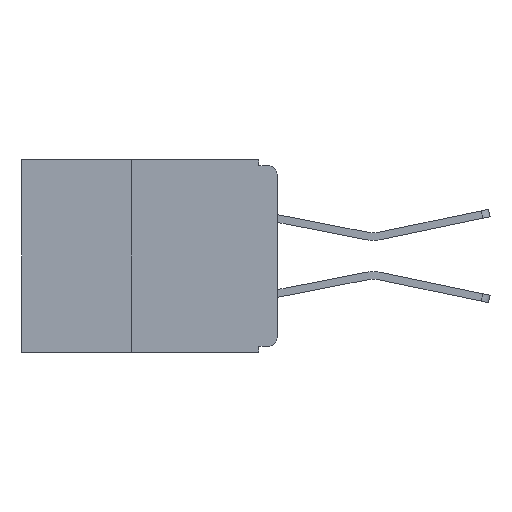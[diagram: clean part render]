
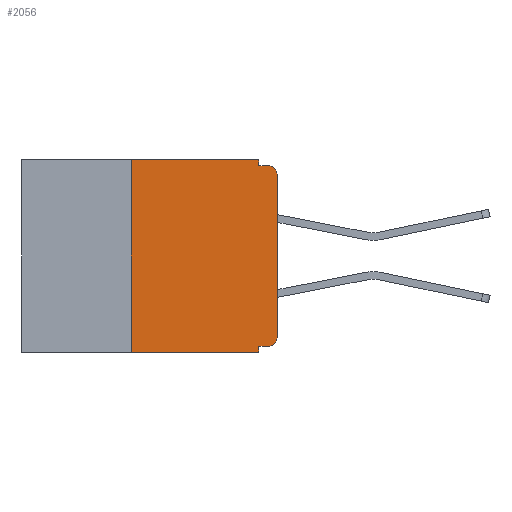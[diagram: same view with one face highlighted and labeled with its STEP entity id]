
A CAD part, left-side view. The second image highlights one B-rep face of the part: STEP entity #2056.
In plain terms, the highlighted planar face has unit normal (-1, 0, 0).
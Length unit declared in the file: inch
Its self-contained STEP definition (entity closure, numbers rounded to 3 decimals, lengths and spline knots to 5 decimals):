
#40 = CARTESIAN_POINT ( 'NONE',  ( 0., 0.031, -0.32 ) ) ;
#153 = PLANE ( 'NONE',  #12464 ) ;
#538 = CARTESIAN_POINT ( 'NONE',  ( 0., 0., -0.025 ) ) ;
#585 = VERTEX_POINT ( 'NONE', #9970 ) ;
#678 = FACE_OUTER_BOUND ( 'NONE', #1296, .T. ) ;
#698 = VERTEX_POINT ( 'NONE', #15077 ) ;
#737 = ORIENTED_EDGE ( 'NONE', *, *, #8602, .F. ) ;
#1296 = EDGE_LOOP ( 'NONE', ( #13047, #6669, #3337, #14730, #11552, #10808, #3109, #10611, #737, #13391 ) ) ;
#1690 = VECTOR ( 'NONE', #10658, 39.37008 ) ;
#1856 = LINE ( 'NONE', #3716, #8079 ) ;
#2025 = DIRECTION ( 'NONE',  ( 0., 0., -1. ) ) ;
#2056 = ADVANCED_FACE ( 'NONE', ( #678 ), #153, .F. ) ;
#2126 = DIRECTION ( 'NONE',  ( 0., 1., 0. ) ) ;
#2151 = LINE ( 'NONE', #2395, #14745 ) ;
#2202 = LINE ( 'NONE', #5882, #8791 ) ;
#2259 = VERTEX_POINT ( 'NONE', #15441 ) ;
#2395 = CARTESIAN_POINT ( 'NONE',  ( 0., 0., -0.32 ) ) ;
#2409 = EDGE_CURVE ( 'NONE', #6711, #2259, #1856, .T. ) ;
#2489 = EDGE_CURVE ( 'NONE', #698, #13490, #10160, .T. ) ;
#2504 = DIRECTION ( 'NONE',  ( 0., -1., 0. ) ) ;
#2893 = VECTOR ( 'NONE', #7221, 39.37008 ) ;
#2975 = DIRECTION ( 'NONE',  ( 0., -1., 0. ) ) ;
#3023 = CARTESIAN_POINT ( 'NONE',  ( 0., 0.437, -0.33 ) ) ;
#3027 = CARTESIAN_POINT ( 'NONE',  ( 0., 0.437, 0. ) ) ;
#3109 = ORIENTED_EDGE ( 'NONE', *, *, #6402, .T. ) ;
#3196 = CARTESIAN_POINT ( 'NONE',  ( 0., 0.25, 0. ) ) ;
#3272 = CARTESIAN_POINT ( 'NONE',  ( 0., 0.25, -0.33 ) ) ;
#3337 = ORIENTED_EDGE ( 'NONE', *, *, #2489, .F. ) ;
#3424 = VERTEX_POINT ( 'NONE', #8986 ) ;
#3522 = VECTOR ( 'NONE', #2975, 39.37008 ) ;
#3716 = CARTESIAN_POINT ( 'NONE',  ( 0., 0.031, -0.33 ) ) ;
#3822 = VERTEX_POINT ( 'NONE', #3272 ) ;
#4166 = DIRECTION ( 'NONE',  ( 0., -1., 0. ) ) ;
#4202 = CARTESIAN_POINT ( 'NONE',  ( 0., 0.437, 0. ) ) ;
#4497 = EDGE_CURVE ( 'NONE', #8706, #13490, #12151, .T. ) ;
#4676 = VERTEX_POINT ( 'NONE', #12878 ) ;
#5375 = CARTESIAN_POINT ( 'NONE',  ( 0., 0., -0.01 ) ) ;
#5882 = CARTESIAN_POINT ( 'NONE',  ( 0., 0.031, 0. ) ) ;
#6402 = EDGE_CURVE ( 'NONE', #3822, #2259, #7008, .T. ) ;
#6669 = ORIENTED_EDGE ( 'NONE', *, *, #4497, .T. ) ;
#6711 = VERTEX_POINT ( 'NONE', #40 ) ;
#7008 = LINE ( 'NONE', #3023, #3522 ) ;
#7221 = DIRECTION ( 'NONE',  ( 0., 0., 1. ) ) ;
#7328 = VECTOR ( 'NONE', #2504, 39.37008 ) ;
#7342 = CARTESIAN_POINT ( 'NONE',  ( 0., 0.25, -0.33 ) ) ;
#7368 = AXIS2_PLACEMENT_3D ( 'NONE', #11338, #12132, #10103 ) ;
#7424 = VERTEX_POINT ( 'NONE', #3196 ) ;
#7740 = VECTOR ( 'NONE', #4166, 39.37008 ) ;
#7812 = DIRECTION ( 'NONE',  ( -1., 0., 0. ) ) ;
#7815 = DIRECTION ( 'NONE',  ( 0., 0., -1. ) ) ;
#7915 = CARTESIAN_POINT ( 'NONE',  ( 0., 0.015, -0.305 ) ) ;
#8079 = VECTOR ( 'NONE', #8784, 39.37008 ) ;
#8312 = LINE ( 'NONE', #13029, #1690 ) ;
#8387 = EDGE_CURVE ( 'NONE', #585, #4676, #15092, .T. ) ;
#8602 = EDGE_CURVE ( 'NONE', #585, #6711, #2151, .T. ) ;
#8706 = VERTEX_POINT ( 'NONE', #538 ) ;
#8784 = DIRECTION ( 'NONE',  ( 0., 0., -1. ) ) ;
#8791 = VECTOR ( 'NONE', #14285, 39.37008 ) ;
#8986 = CARTESIAN_POINT ( 'NONE',  ( 0., 0.031, 0. ) ) ;
#9407 = AXIS2_PLACEMENT_3D ( 'NONE', #7915, #7812, #7815 ) ;
#9827 = EDGE_CURVE ( 'NONE', #3822, #7424, #15818, .T. ) ;
#9970 = CARTESIAN_POINT ( 'NONE',  ( 0., 0.015, -0.32 ) ) ;
#10103 = DIRECTION ( 'NONE',  ( 0., 0., -1. ) ) ;
#10160 = LINE ( 'NONE', #5375, #7328 ) ;
#10194 = EDGE_CURVE ( 'NONE', #7424, #3424, #14113, .T. ) ;
#10611 = ORIENTED_EDGE ( 'NONE', *, *, #2409, .F. ) ;
#10658 = DIRECTION ( 'NONE',  ( 0., 0., 1. ) ) ;
#10808 = ORIENTED_EDGE ( 'NONE', *, *, #9827, .F. ) ;
#11338 = CARTESIAN_POINT ( 'NONE',  ( 0., 0.015, -0.025 ) ) ;
#11552 = ORIENTED_EDGE ( 'NONE', *, *, #10194, .F. ) ;
#12132 = DIRECTION ( 'NONE',  ( -1., 0., 0. ) ) ;
#12151 = CIRCLE ( 'NONE', #7368, 0.015 ) ;
#12464 = AXIS2_PLACEMENT_3D ( 'NONE', #3027, #15137, #2025 ) ;
#12708 = EDGE_CURVE ( 'NONE', #3424, #698, #2202, .T. ) ;
#12797 = CARTESIAN_POINT ( 'NONE',  ( 0., 0.015, -0.01 ) ) ;
#12878 = CARTESIAN_POINT ( 'NONE',  ( 0., 0., -0.305 ) ) ;
#13029 = CARTESIAN_POINT ( 'NONE',  ( 0., 0., 0. ) ) ;
#13047 = ORIENTED_EDGE ( 'NONE', *, *, #14731, .T. ) ;
#13391 = ORIENTED_EDGE ( 'NONE', *, *, #8387, .T. ) ;
#13490 = VERTEX_POINT ( 'NONE', #12797 ) ;
#14113 = LINE ( 'NONE', #4202, #7740 ) ;
#14285 = DIRECTION ( 'NONE',  ( 0., 0., -1. ) ) ;
#14730 = ORIENTED_EDGE ( 'NONE', *, *, #12708, .F. ) ;
#14731 = EDGE_CURVE ( 'NONE', #4676, #8706, #8312, .T. ) ;
#14745 = VECTOR ( 'NONE', #2126, 39.37008 ) ;
#15077 = CARTESIAN_POINT ( 'NONE',  ( 0., 0.031, -0.01 ) ) ;
#15092 = CIRCLE ( 'NONE', #9407, 0.015 ) ;
#15137 = DIRECTION ( 'NONE',  ( 1., 0., 0. ) ) ;
#15441 = CARTESIAN_POINT ( 'NONE',  ( 0., 0.031, -0.33 ) ) ;
#15818 = LINE ( 'NONE', #7342, #2893 ) ;
